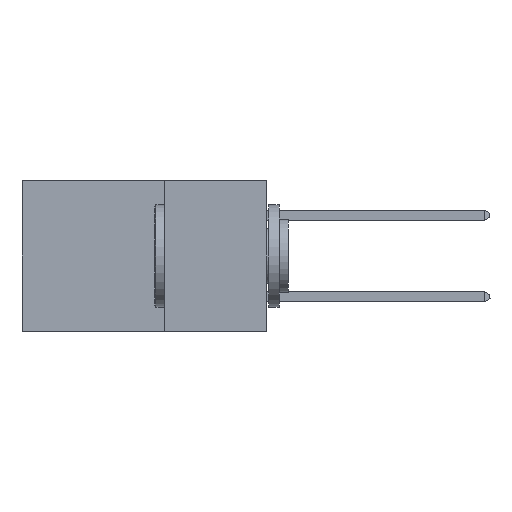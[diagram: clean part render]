
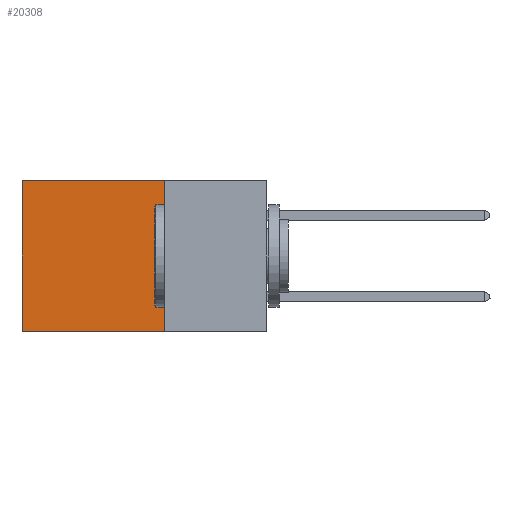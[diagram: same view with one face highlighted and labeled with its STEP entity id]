
A CAD part, left-side view. The second image highlights one B-rep face of the part: STEP entity #20308.
In plain terms, the highlighted planar face has unit normal (-1, 0, 0).
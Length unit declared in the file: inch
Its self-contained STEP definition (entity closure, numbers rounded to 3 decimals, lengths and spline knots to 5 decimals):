
#373 = EDGE_CURVE ( 'NONE', #20155, #6767, #6157, .T. ) ;
#1074 = EDGE_CURVE ( 'NONE', #2687, #1810, #14844, .T. ) ;
#1401 = DIRECTION ( 'NONE',  ( 0., 0., -1. ) ) ;
#1810 = VERTEX_POINT ( 'NONE', #9817 ) ;
#1813 = LINE ( 'NONE', #11930, #7121 ) ;
#2687 = VERTEX_POINT ( 'NONE', #6172 ) ;
#4231 = ORIENTED_EDGE ( 'NONE', *, *, #5050, .F. ) ;
#4380 = CARTESIAN_POINT ( 'NONE',  ( 0.2875, 0.25, 0. ) ) ;
#4659 = PLANE ( 'NONE',  #20296 ) ;
#5050 = EDGE_CURVE ( 'NONE', #6767, #1810, #1813, .T. ) ;
#5089 = VECTOR ( 'NONE', #18389, 39.37008 ) ;
#6157 = LINE ( 'NONE', #6307, #5089 ) ;
#6172 = CARTESIAN_POINT ( 'NONE',  ( 0.2875, 0.6, 0. ) ) ;
#6307 = CARTESIAN_POINT ( 'NONE',  ( 0.2875, 0.25, 0. ) ) ;
#6767 = VERTEX_POINT ( 'NONE', #11868 ) ;
#6992 = DIRECTION ( 'NONE',  ( 0., 1., 0. ) ) ;
#7121 = VECTOR ( 'NONE', #6992, 39.37008 ) ;
#9060 = CARTESIAN_POINT ( 'NONE',  ( 0.2875, 0.6, 0. ) ) ;
#9817 = CARTESIAN_POINT ( 'NONE',  ( 0.2875, 0.6, -0.37 ) ) ;
#11412 = EDGE_CURVE ( 'NONE', #20155, #2687, #13068, .T. ) ;
#11644 = ORIENTED_EDGE ( 'NONE', *, *, #11412, .T. ) ;
#11868 = CARTESIAN_POINT ( 'NONE',  ( 0.2875, 0.25, -0.37 ) ) ;
#11930 = CARTESIAN_POINT ( 'NONE',  ( 0.2875, 0.25, -0.37 ) ) ;
#13068 = LINE ( 'NONE', #14804, #13611 ) ;
#13611 = VECTOR ( 'NONE', #15227, 39.37008 ) ;
#14804 = CARTESIAN_POINT ( 'NONE',  ( 0.2875, 0.25, 0. ) ) ;
#14844 = LINE ( 'NONE', #9060, #21211 ) ;
#15227 = DIRECTION ( 'NONE',  ( 0., 1., 0. ) ) ;
#18089 = EDGE_LOOP ( 'NONE', ( #21703, #4231, #20096, #11644 ) ) ;
#18389 = DIRECTION ( 'NONE',  ( 0., 0., -1. ) ) ;
#18966 = DIRECTION ( 'NONE',  ( 0., 0., -1. ) ) ;
#19492 = FACE_OUTER_BOUND ( 'NONE', #18089, .T. ) ;
#20048 = CARTESIAN_POINT ( 'NONE',  ( 0.2875, 0.25, 0. ) ) ;
#20096 = ORIENTED_EDGE ( 'NONE', *, *, #373, .F. ) ;
#20155 = VERTEX_POINT ( 'NONE', #4380 ) ;
#20296 = AXIS2_PLACEMENT_3D ( 'NONE', #20048, #21754, #1401 ) ;
#20308 = ADVANCED_FACE ( 'NONE', ( #19492 ), #4659, .F. ) ;
#21211 = VECTOR ( 'NONE', #18966, 39.37008 ) ;
#21703 = ORIENTED_EDGE ( 'NONE', *, *, #1074, .T. ) ;
#21754 = DIRECTION ( 'NONE',  ( 1., 0., 0. ) ) ;
